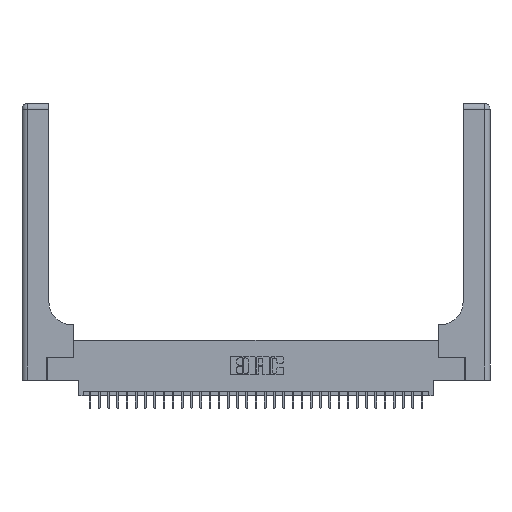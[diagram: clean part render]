
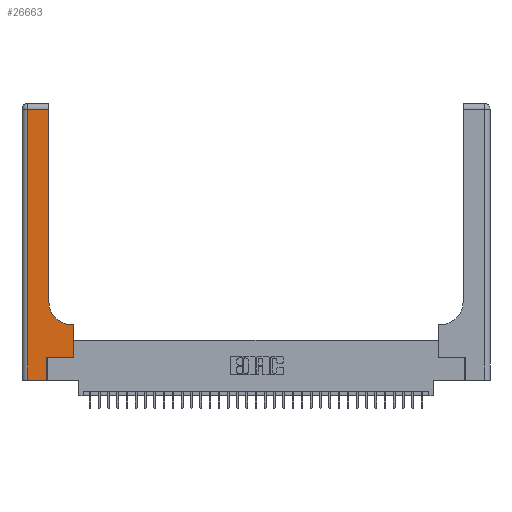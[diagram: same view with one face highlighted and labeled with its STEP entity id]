
A CAD part, top view. The second image highlights one B-rep face of the part: STEP entity #26663.
In plain terms, the highlighted planar face has unit normal (0, 0, 1).
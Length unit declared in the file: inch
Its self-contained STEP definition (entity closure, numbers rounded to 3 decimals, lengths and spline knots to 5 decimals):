
#656 = VERTEX_POINT ( 'NONE', #22661 ) ;
#1183 = CIRCLE ( 'NONE', #6872, 0.25 ) ;
#1294 = CARTESIAN_POINT ( 'NONE',  ( 0., 2.94, 0.37 ) ) ;
#2039 = ORIENTED_EDGE ( 'NONE', *, *, #9086, .T. ) ;
#2522 = EDGE_CURVE ( 'NONE', #12887, #20739, #8152, .T. ) ;
#3165 = DIRECTION ( 'NONE',  ( 0., 1., 0. ) ) ;
#3311 = ORIENTED_EDGE ( 'NONE', *, *, #4719, .T. ) ;
#3691 = LINE ( 'NONE', #23078, #27625 ) ;
#4719 = EDGE_CURVE ( 'NONE', #11791, #26019, #9643, .T. ) ;
#4728 = CARTESIAN_POINT ( 'NONE',  ( 0., 3., 0.37 ) ) ;
#5602 = VERTEX_POINT ( 'NONE', #15564 ) ;
#5985 = CARTESIAN_POINT ( 'NONE',  ( 0.06, 3., 0.37 ) ) ;
#6307 = CARTESIAN_POINT ( 'NONE',  ( 0.2915, 0.6, 0.37 ) ) ;
#6339 = DIRECTION ( 'NONE',  ( 0., -1., 0. ) ) ;
#6541 = DIRECTION ( 'NONE',  ( 0., 0., -1. ) ) ;
#6872 = AXIS2_PLACEMENT_3D ( 'NONE', #11888, #6541, #22383 ) ;
#7928 = VERTEX_POINT ( 'NONE', #15554 ) ;
#7981 = CARTESIAN_POINT ( 'NONE',  ( 0.5585, 0.25, 0.37 ) ) ;
#8152 = LINE ( 'NONE', #19014, #29302 ) ;
#8903 = ORIENTED_EDGE ( 'NONE', *, *, #33895, .T. ) ;
#8998 = VERTEX_POINT ( 'NONE', #33034 ) ;
#9086 = EDGE_CURVE ( 'NONE', #8998, #17832, #1183, .T. ) ;
#9168 = VECTOR ( 'NONE', #14445, 39.37008 ) ;
#9315 = LINE ( 'NONE', #6307, #23879 ) ;
#9566 = ORIENTED_EDGE ( 'NONE', *, *, #26994, .T. ) ;
#9643 = LINE ( 'NONE', #1294, #11227 ) ;
#9873 = DIRECTION ( 'NONE',  ( 0., 0., -1. ) ) ;
#11015 = LINE ( 'NONE', #21879, #27047 ) ;
#11207 = CARTESIAN_POINT ( 'NONE',  ( 0.269, 0.25, 0.37 ) ) ;
#11227 = VECTOR ( 'NONE', #28491, 39.37008 ) ;
#11791 = VERTEX_POINT ( 'NONE', #21903 ) ;
#11888 = CARTESIAN_POINT ( 'NONE',  ( 0.5415, 0.85, 0.37 ) ) ;
#12679 = ORIENTED_EDGE ( 'NONE', *, *, #2522, .T. ) ;
#12887 = VERTEX_POINT ( 'NONE', #26015 ) ;
#14288 = EDGE_CURVE ( 'NONE', #20739, #5602, #22447, .T. ) ;
#14445 = DIRECTION ( 'NONE',  ( 1., 0., 0. ) ) ;
#14495 = DIRECTION ( 'NONE',  ( -1., 0., 0. ) ) ;
#15234 = ORIENTED_EDGE ( 'NONE', *, *, #22601, .T. ) ;
#15554 = CARTESIAN_POINT ( 'NONE',  ( 0.5585, 0.6, 0.37 ) ) ;
#15564 = CARTESIAN_POINT ( 'NONE',  ( 0.5585, 0.25, 0.37 ) ) ;
#15575 = DIRECTION ( 'NONE',  ( -1., 0., 0. ) ) ;
#15751 = PLANE ( 'NONE',  #18190 ) ;
#16927 = EDGE_LOOP ( 'NONE', ( #15234, #3311, #22903, #8903, #12679, #19133, #18450, #9566, #2039 ) ) ;
#17212 = DIRECTION ( 'NONE',  ( 0., 1., 0. ) ) ;
#17832 = VERTEX_POINT ( 'NONE', #28082 ) ;
#18190 = AXIS2_PLACEMENT_3D ( 'NONE', #4728, #9873, #15575 ) ;
#18450 = ORIENTED_EDGE ( 'NONE', *, *, #27397, .T. ) ;
#19014 = CARTESIAN_POINT ( 'NONE',  ( 0.269, 0., 0.37 ) ) ;
#19133 = ORIENTED_EDGE ( 'NONE', *, *, #14288, .T. ) ;
#20303 = VECTOR ( 'NONE', #6339, 39.37008 ) ;
#20739 = VERTEX_POINT ( 'NONE', #11207 ) ;
#21213 = CARTESIAN_POINT ( 'NONE',  ( 0.06, 2.94, 0.37 ) ) ;
#21872 = DIRECTION ( 'NONE',  ( 0., 1., 0. ) ) ;
#21879 = CARTESIAN_POINT ( 'NONE',  ( 0., 0., 0.37 ) ) ;
#21903 = CARTESIAN_POINT ( 'NONE',  ( 0.2915, 2.94, 0.37 ) ) ;
#22383 = DIRECTION ( 'NONE',  ( 1., 0., 0. ) ) ;
#22447 = LINE ( 'NONE', #25457, #9168 ) ;
#22601 = EDGE_CURVE ( 'NONE', #17832, #11791, #3691, .T. ) ;
#22661 = CARTESIAN_POINT ( 'NONE',  ( 0.06, 0., 0.37 ) ) ;
#22903 = ORIENTED_EDGE ( 'NONE', *, *, #25308, .T. ) ;
#23078 = CARTESIAN_POINT ( 'NONE',  ( 0.2915, 3., 0.37 ) ) ;
#23879 = VECTOR ( 'NONE', #14495, 39.37008 ) ;
#24018 = VECTOR ( 'NONE', #3165, 39.37008 ) ;
#25308 = EDGE_CURVE ( 'NONE', #26019, #656, #30864, .T. ) ;
#25457 = CARTESIAN_POINT ( 'NONE',  ( 0.269, 0.25, 0.37 ) ) ;
#26015 = CARTESIAN_POINT ( 'NONE',  ( 0.269, 0., 0.37 ) ) ;
#26019 = VERTEX_POINT ( 'NONE', #21213 ) ;
#26663 = ADVANCED_FACE ( 'NONE', ( #29073 ), #15751, .F. ) ;
#26994 = EDGE_CURVE ( 'NONE', #7928, #8998, #9315, .T. ) ;
#27047 = VECTOR ( 'NONE', #30038, 39.37008 ) ;
#27397 = EDGE_CURVE ( 'NONE', #5602, #7928, #32335, .T. ) ;
#27625 = VECTOR ( 'NONE', #17212, 39.37008 ) ;
#28082 = CARTESIAN_POINT ( 'NONE',  ( 0.2915, 0.85, 0.37 ) ) ;
#28491 = DIRECTION ( 'NONE',  ( -1., 0., 0. ) ) ;
#29073 = FACE_OUTER_BOUND ( 'NONE', #16927, .T. ) ;
#29302 = VECTOR ( 'NONE', #21872, 39.37008 ) ;
#30038 = DIRECTION ( 'NONE',  ( 1., 0., 0. ) ) ;
#30864 = LINE ( 'NONE', #5985, #20303 ) ;
#32335 = LINE ( 'NONE', #7981, #24018 ) ;
#33034 = CARTESIAN_POINT ( 'NONE',  ( 0.5415, 0.6, 0.37 ) ) ;
#33895 = EDGE_CURVE ( 'NONE', #656, #12887, #11015, .T. ) ;
